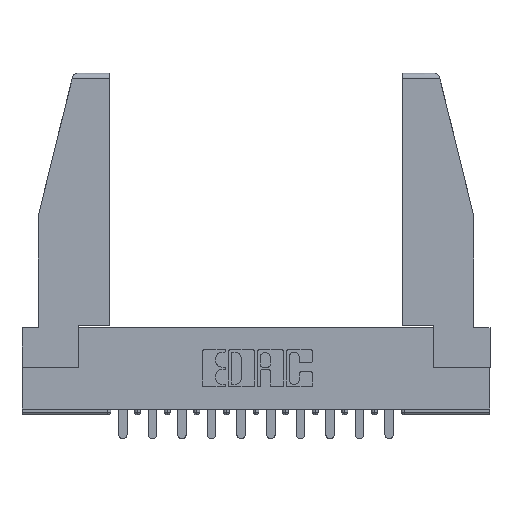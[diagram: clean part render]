
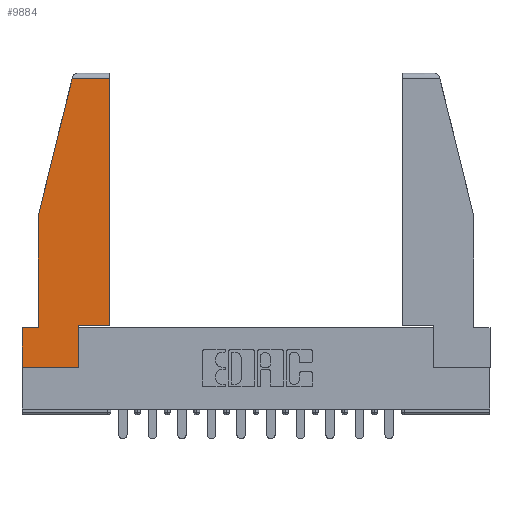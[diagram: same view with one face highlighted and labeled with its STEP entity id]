
A CAD part, top view. The second image highlights one B-rep face of the part: STEP entity #9884.
In plain terms, the highlighted planar face has unit normal (0, 0, 1).
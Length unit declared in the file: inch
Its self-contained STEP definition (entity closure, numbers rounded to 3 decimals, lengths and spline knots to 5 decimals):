
#86 = ORIENTED_EDGE ( 'NONE', *, *, #6538, .T. ) ;
#150 = CARTESIAN_POINT ( 'NONE',  ( 0.271, 1.55, 0. ) ) ;
#620 = DIRECTION ( 'NONE',  ( 1., 0., 0. ) ) ;
#698 = CARTESIAN_POINT ( 'NONE',  ( 0.461, 1.52, 0. ) ) ;
#756 = FACE_OUTER_BOUND ( 'NONE', #11161, .T. ) ;
#866 = DIRECTION ( 'NONE',  ( -1., 0., 0. ) ) ;
#1037 = VECTOR ( 'NONE', #866, 39.37008 ) ;
#1072 = DIRECTION ( 'NONE',  ( -1., 0., 0. ) ) ;
#1196 = EDGE_CURVE ( 'NONE', #14712, #8605, #13947, .T. ) ;
#1198 = CARTESIAN_POINT ( 'NONE',  ( 0.297, 0.223, 0. ) ) ;
#1367 = DIRECTION ( 'NONE',  ( 0., -1., 0. ) ) ;
#1381 = CARTESIAN_POINT ( 'NONE',  ( 0.297, 0.223, 0. ) ) ;
#1760 = EDGE_CURVE ( 'NONE', #2603, #2439, #8210, .T. ) ;
#1776 = VECTOR ( 'NONE', #3889, 39.37008 ) ;
#1780 = VERTEX_POINT ( 'NONE', #6544 ) ;
#1886 = LINE ( 'NONE', #11872, #14865 ) ;
#2423 = EDGE_CURVE ( 'NONE', #12532, #14593, #2789, .T. ) ;
#2439 = VERTEX_POINT ( 'NONE', #1381 ) ;
#2574 = PLANE ( 'NONE',  #4750 ) ;
#2603 = VERTEX_POINT ( 'NONE', #10026 ) ;
#2619 = LINE ( 'NONE', #13481, #5703 ) ;
#2789 = LINE ( 'NONE', #13072, #14727 ) ;
#3889 = DIRECTION ( 'NONE',  ( 0., 1., 0. ) ) ;
#3892 = DIRECTION ( 'NONE',  ( 0., 0., 1. ) ) ;
#4412 = LINE ( 'NONE', #1198, #9583 ) ;
#4750 = AXIS2_PLACEMENT_3D ( 'NONE', #16947, #3892, #13096 ) ;
#4780 = ORIENTED_EDGE ( 'NONE', *, *, #16724, .T. ) ;
#4837 = CARTESIAN_POINT ( 'NONE',  ( 0.461, 0.223, 0. ) ) ;
#5193 = ORIENTED_EDGE ( 'NONE', *, *, #7269, .T. ) ;
#5703 = VECTOR ( 'NONE', #620, 39.37008 ) ;
#6008 = CARTESIAN_POINT ( 'NONE',  ( 0., 0.21, 0. ) ) ;
#6242 = VERTEX_POINT ( 'NONE', #6356 ) ;
#6356 = CARTESIAN_POINT ( 'NONE',  ( 0.086, 0.8, 0. ) ) ;
#6435 = CARTESIAN_POINT ( 'NONE',  ( 0.086, 0.21, 0. ) ) ;
#6538 = EDGE_CURVE ( 'NONE', #6242, #16739, #1886, .T. ) ;
#6544 = CARTESIAN_POINT ( 'NONE',  ( 0.2636, 1.52, 0. ) ) ;
#6773 = LINE ( 'NONE', #150, #16830 ) ;
#7046 = CARTESIAN_POINT ( 'NONE',  ( 0.461, 0.223, 0. ) ) ;
#7269 = EDGE_CURVE ( 'NONE', #8605, #1780, #11759, .T. ) ;
#7451 = CARTESIAN_POINT ( 'NONE',  ( 0., 1.52, 0. ) ) ;
#8210 = LINE ( 'NONE', #14369, #1776 ) ;
#8605 = VERTEX_POINT ( 'NONE', #698 ) ;
#9204 = ORIENTED_EDGE ( 'NONE', *, *, #16423, .T. ) ;
#9406 = DIRECTION ( 'NONE',  ( -0.239, -0.971, 0. ) ) ;
#9583 = VECTOR ( 'NONE', #10413, 39.37008 ) ;
#9789 = EDGE_CURVE ( 'NONE', #14593, #2603, #2619, .T. ) ;
#9884 = ADVANCED_FACE ( 'NONE', ( #756 ), #2574, .T. ) ;
#10026 = CARTESIAN_POINT ( 'NONE',  ( 0.297, 0., 0. ) ) ;
#10237 = VECTOR ( 'NONE', #13818, 39.37008 ) ;
#10413 = DIRECTION ( 'NONE',  ( 1., 0., 0. ) ) ;
#10448 = VECTOR ( 'NONE', #1072, 39.37008 ) ;
#11161 = EDGE_LOOP ( 'NONE', ( #12477, #5193, #9204, #86, #4780, #15952, #12066, #11237, #15305 ) ) ;
#11237 = ORIENTED_EDGE ( 'NONE', *, *, #1760, .T. ) ;
#11759 = LINE ( 'NONE', #7451, #1037 ) ;
#11872 = CARTESIAN_POINT ( 'NONE',  ( 0.086, 0.8, 0. ) ) ;
#12066 = ORIENTED_EDGE ( 'NONE', *, *, #9789, .T. ) ;
#12477 = ORIENTED_EDGE ( 'NONE', *, *, #1196, .T. ) ;
#12532 = VERTEX_POINT ( 'NONE', #6008 ) ;
#12791 = CARTESIAN_POINT ( 'NONE',  ( 0., 0., 0. ) ) ;
#13037 = EDGE_CURVE ( 'NONE', #2439, #14712, #4412, .T. ) ;
#13072 = CARTESIAN_POINT ( 'NONE',  ( 0., 0.21, 0. ) ) ;
#13096 = DIRECTION ( 'NONE',  ( 1., 0., 0. ) ) ;
#13177 = DIRECTION ( 'NONE',  ( 0., -1., 0. ) ) ;
#13319 = LINE ( 'NONE', #16891, #10448 ) ;
#13481 = CARTESIAN_POINT ( 'NONE',  ( 0., 0., 0. ) ) ;
#13818 = DIRECTION ( 'NONE',  ( 0., 1., 0. ) ) ;
#13947 = LINE ( 'NONE', #7046, #10237 ) ;
#14369 = CARTESIAN_POINT ( 'NONE',  ( 0.297, 0., 0. ) ) ;
#14593 = VERTEX_POINT ( 'NONE', #12791 ) ;
#14712 = VERTEX_POINT ( 'NONE', #4837 ) ;
#14727 = VECTOR ( 'NONE', #13177, 39.37008 ) ;
#14865 = VECTOR ( 'NONE', #1367, 39.37008 ) ;
#15305 = ORIENTED_EDGE ( 'NONE', *, *, #13037, .T. ) ;
#15952 = ORIENTED_EDGE ( 'NONE', *, *, #2423, .T. ) ;
#16423 = EDGE_CURVE ( 'NONE', #1780, #6242, #6773, .T. ) ;
#16724 = EDGE_CURVE ( 'NONE', #16739, #12532, #13319, .T. ) ;
#16739 = VERTEX_POINT ( 'NONE', #6435 ) ;
#16830 = VECTOR ( 'NONE', #9406, 39.37008 ) ;
#16891 = CARTESIAN_POINT ( 'NONE',  ( 0., 0.21, 0. ) ) ;
#16947 = CARTESIAN_POINT ( 'NONE',  ( 0., 0., 0. ) ) ;
